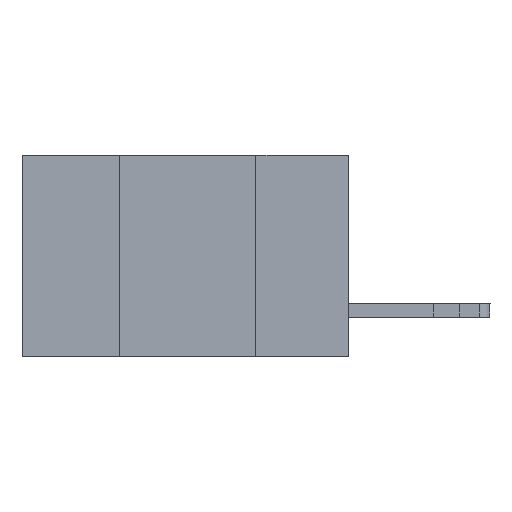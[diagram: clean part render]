
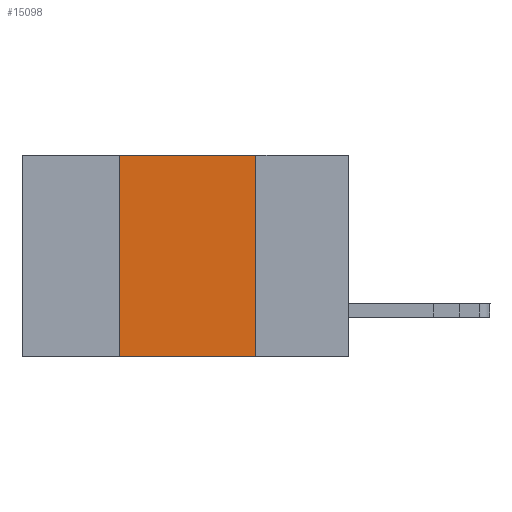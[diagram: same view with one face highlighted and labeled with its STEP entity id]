
A CAD part, left-side view. The second image highlights one B-rep face of the part: STEP entity #15098.
In plain terms, the highlighted planar face has unit normal (-1, 0, 0).
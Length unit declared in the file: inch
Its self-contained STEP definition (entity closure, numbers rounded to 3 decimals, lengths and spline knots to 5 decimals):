
#104 = CARTESIAN_POINT ( 'NONE',  ( 0., 0.6, -0.37 ) ) ;
#508 = LINE ( 'NONE', #604, #17655 ) ;
#604 = CARTESIAN_POINT ( 'NONE',  ( 0., 0.42, 0. ) ) ;
#667 = AXIS2_PLACEMENT_3D ( 'NONE', #2613, #4444, #959 ) ;
#959 = DIRECTION ( 'NONE',  ( 0., 0., -1. ) ) ;
#2466 = DIRECTION ( 'NONE',  ( 0., 0., 1. ) ) ;
#2613 = CARTESIAN_POINT ( 'NONE',  ( 0., 0.6, 0. ) ) ;
#2881 = VECTOR ( 'NONE', #4727, 39.37008 ) ;
#4444 = DIRECTION ( 'NONE',  ( 1., 0., 0. ) ) ;
#4727 = DIRECTION ( 'NONE',  ( 0., 0., -1. ) ) ;
#6463 = ORIENTED_EDGE ( 'NONE', *, *, #8182, .F. ) ;
#6726 = CARTESIAN_POINT ( 'NONE',  ( 0., 0.17, 0. ) ) ;
#6884 = ORIENTED_EDGE ( 'NONE', *, *, #19495, .F. ) ;
#7707 = PLANE ( 'NONE',  #667 ) ;
#8056 = LINE ( 'NONE', #104, #10895 ) ;
#8093 = CARTESIAN_POINT ( 'NONE',  ( 0., 0.17, 0. ) ) ;
#8182 = EDGE_CURVE ( 'NONE', #16366, #16461, #9872, .T. ) ;
#8686 = VERTEX_POINT ( 'NONE', #12208 ) ;
#9872 = LINE ( 'NONE', #18446, #15239 ) ;
#9877 = ORIENTED_EDGE ( 'NONE', *, *, #19787, .F. ) ;
#10895 = VECTOR ( 'NONE', #11653, 39.37008 ) ;
#10932 = EDGE_LOOP ( 'NONE', ( #9877, #6463, #6884, #16678 ) ) ;
#11653 = DIRECTION ( 'NONE',  ( 0., -1., 0. ) ) ;
#12208 = CARTESIAN_POINT ( 'NONE',  ( 0., 0.17, -0.37 ) ) ;
#15098 = ADVANCED_FACE ( 'NONE', ( #19527 ), #7707, .F. ) ;
#15239 = VECTOR ( 'NONE', #21463, 39.37008 ) ;
#16366 = VERTEX_POINT ( 'NONE', #16498 ) ;
#16461 = VERTEX_POINT ( 'NONE', #6726 ) ;
#16498 = CARTESIAN_POINT ( 'NONE',  ( 0., 0.42, 0. ) ) ;
#16678 = ORIENTED_EDGE ( 'NONE', *, *, #20492, .T. ) ;
#17655 = VECTOR ( 'NONE', #2466, 39.37008 ) ;
#17733 = VERTEX_POINT ( 'NONE', #18458 ) ;
#18446 = CARTESIAN_POINT ( 'NONE',  ( 0., 0.6, 0. ) ) ;
#18458 = CARTESIAN_POINT ( 'NONE',  ( 0., 0.42, -0.37 ) ) ;
#19495 = EDGE_CURVE ( 'NONE', #17733, #16366, #508, .T. ) ;
#19527 = FACE_OUTER_BOUND ( 'NONE', #10932, .T. ) ;
#19787 = EDGE_CURVE ( 'NONE', #16461, #8686, #20029, .T. ) ;
#20029 = LINE ( 'NONE', #8093, #2881 ) ;
#20492 = EDGE_CURVE ( 'NONE', #17733, #8686, #8056, .T. ) ;
#21463 = DIRECTION ( 'NONE',  ( 0., -1., 0. ) ) ;
